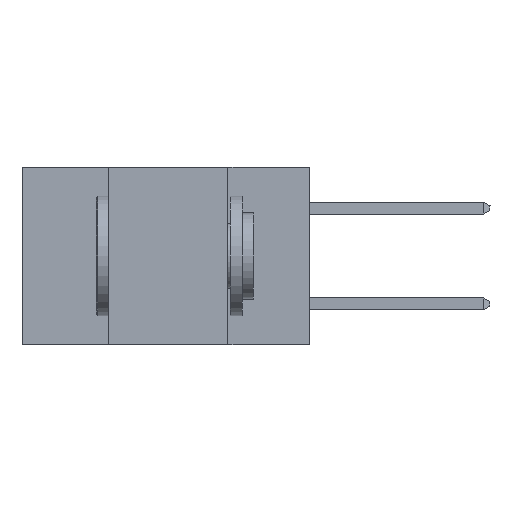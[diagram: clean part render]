
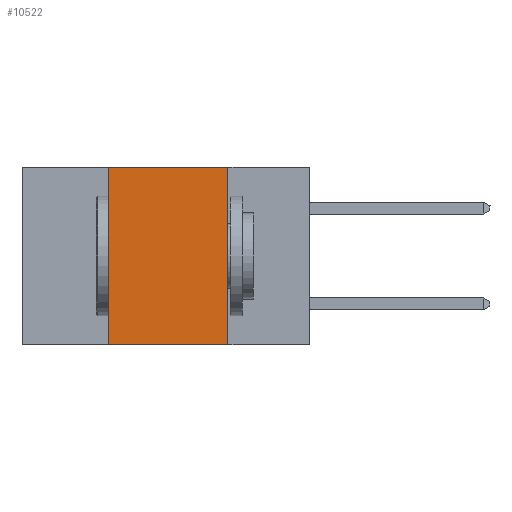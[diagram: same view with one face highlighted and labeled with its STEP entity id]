
A CAD part, left-side view. The second image highlights one B-rep face of the part: STEP entity #10522.
In plain terms, the highlighted planar face has unit normal (-1, 0, 0).
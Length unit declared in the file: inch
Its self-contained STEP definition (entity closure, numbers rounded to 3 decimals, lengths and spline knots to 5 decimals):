
#657 = AXIS2_PLACEMENT_3D ( 'NONE', #13117, #2590, #8957 ) ;
#1360 = VERTEX_POINT ( 'NONE', #4029 ) ;
#1905 = DIRECTION ( 'NONE',  ( 0., -1., 0. ) ) ;
#2203 = VECTOR ( 'NONE', #1905, 39.37008 ) ;
#2422 = ORIENTED_EDGE ( 'NONE', *, *, #5686, .F. ) ;
#2590 = DIRECTION ( 'NONE',  ( 1., 0., 0. ) ) ;
#2686 = CARTESIAN_POINT ( 'NONE',  ( 0., 0.17, 0. ) ) ;
#2787 = ORIENTED_EDGE ( 'NONE', *, *, #12815, .T. ) ;
#2883 = LINE ( 'NONE', #13300, #2203 ) ;
#3442 = CARTESIAN_POINT ( 'NONE',  ( 0., 0.17, 0. ) ) ;
#3690 = EDGE_CURVE ( 'NONE', #6084, #8445, #5471, .T. ) ;
#3709 = EDGE_LOOP ( 'NONE', ( #4130, #7959, #2422, #2787 ) ) ;
#4029 = CARTESIAN_POINT ( 'NONE',  ( 0., 0.42, 0. ) ) ;
#4130 = ORIENTED_EDGE ( 'NONE', *, *, #3690, .F. ) ;
#5471 = LINE ( 'NONE', #3442, #11247 ) ;
#5686 = EDGE_CURVE ( 'NONE', #9394, #1360, #10826, .T. ) ;
#5927 = LINE ( 'NONE', #6004, #6759 ) ;
#6004 = CARTESIAN_POINT ( 'NONE',  ( 0., 0.6, 0. ) ) ;
#6084 = VERTEX_POINT ( 'NONE', #2686 ) ;
#6461 = CARTESIAN_POINT ( 'NONE',  ( 0., 0.17, -0.37 ) ) ;
#6759 = VECTOR ( 'NONE', #11291, 39.37008 ) ;
#6766 = FACE_OUTER_BOUND ( 'NONE', #3709, .T. ) ;
#7959 = ORIENTED_EDGE ( 'NONE', *, *, #10710, .F. ) ;
#8445 = VERTEX_POINT ( 'NONE', #6461 ) ;
#8909 = CARTESIAN_POINT ( 'NONE',  ( 0., 0.42, -0.37 ) ) ;
#8957 = DIRECTION ( 'NONE',  ( 0., 0., -1. ) ) ;
#9394 = VERTEX_POINT ( 'NONE', #8909 ) ;
#10064 = DIRECTION ( 'NONE',  ( 0., 0., 1. ) ) ;
#10522 = ADVANCED_FACE ( 'NONE', ( #6766 ), #13017, .F. ) ;
#10710 = EDGE_CURVE ( 'NONE', #1360, #6084, #5927, .T. ) ;
#10826 = LINE ( 'NONE', #11099, #12171 ) ;
#11099 = CARTESIAN_POINT ( 'NONE',  ( 0., 0.42, 0. ) ) ;
#11247 = VECTOR ( 'NONE', #12980, 39.37008 ) ;
#11291 = DIRECTION ( 'NONE',  ( 0., -1., 0. ) ) ;
#12171 = VECTOR ( 'NONE', #10064, 39.37008 ) ;
#12815 = EDGE_CURVE ( 'NONE', #9394, #8445, #2883, .T. ) ;
#12980 = DIRECTION ( 'NONE',  ( 0., 0., -1. ) ) ;
#13017 = PLANE ( 'NONE',  #657 ) ;
#13117 = CARTESIAN_POINT ( 'NONE',  ( 0., 0.6, 0. ) ) ;
#13300 = CARTESIAN_POINT ( 'NONE',  ( 0., 0.6, -0.37 ) ) ;
